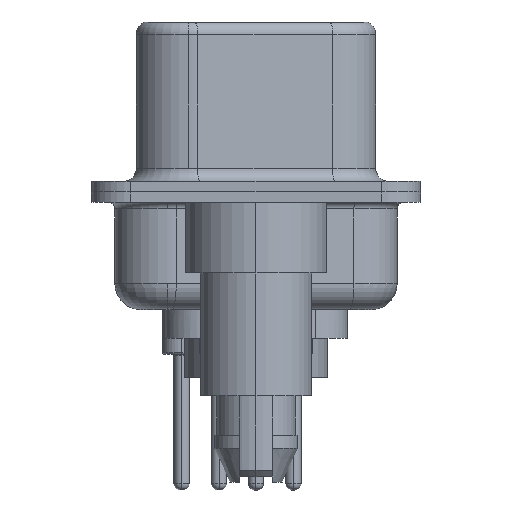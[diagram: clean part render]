
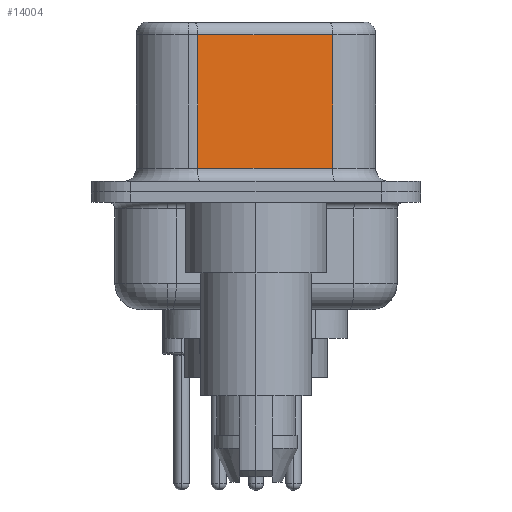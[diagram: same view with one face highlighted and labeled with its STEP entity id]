
A CAD part, left-side view. The second image highlights one B-rep face of the part: STEP entity #14004.
In plain terms, the highlighted planar face has unit normal (-0.985, -0.174, 0).
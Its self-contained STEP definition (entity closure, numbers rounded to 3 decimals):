
#1458 = EDGE_CURVE ( 'NONE', #4819, #14677, #11647, .T. ) ;
#2190 = VERTEX_POINT ( 'NONE', #2467 ) ;
#2467 = CARTESIAN_POINT ( 'NONE',  ( 4.585, -2.927, 0.9 ) ) ;
#2609 = DIRECTION ( 'NONE',  ( -0.174, 0.985, 0. ) ) ;
#2618 = LINE ( 'NONE', #23631, #12493 ) ;
#2813 = EDGE_CURVE ( 'NONE', #15914, #2190, #2618, .T. ) ;
#3540 = VECTOR ( 'NONE', #10122, 1000. ) ;
#4766 = EDGE_CURVE ( 'NONE', #4819, #2190, #15230, .T. ) ;
#4819 = VERTEX_POINT ( 'NONE', #8885 ) ;
#5804 = ORIENTED_EDGE ( 'NONE', *, *, #1458, .T. ) ;
#6627 = LINE ( 'NONE', #10200, #3540 ) ;
#7213 = DIRECTION ( 'NONE',  ( 0.985, 0.174, 0. ) ) ;
#7527 = DIRECTION ( 'NONE',  ( 0.174, -0.985, 0. ) ) ;
#7556 = ORIENTED_EDGE ( 'NONE', *, *, #2813, .T. ) ;
#8885 = CARTESIAN_POINT ( 'NONE',  ( 4.585, -2.927, 6.02 ) ) ;
#9108 = PLANE ( 'NONE',  #25425 ) ;
#9207 = CARTESIAN_POINT ( 'NONE',  ( 4.585, -2.927, 6.52 ) ) ;
#10122 = DIRECTION ( 'NONE',  ( 0., 0., -1. ) ) ;
#10200 = CARTESIAN_POINT ( 'NONE',  ( 3.675, 2.233, 6.52 ) ) ;
#11647 = LINE ( 'NONE', #14417, #18127 ) ;
#12493 = VECTOR ( 'NONE', #7527, 1000. ) ;
#14004 = ADVANCED_FACE ( 'NONE', ( #18443 ), #9108, .F. ) ;
#14287 = CARTESIAN_POINT ( 'NONE',  ( 4.585, -2.927, 6.52 ) ) ;
#14417 = CARTESIAN_POINT ( 'NONE',  ( 4.585, -2.927, 6.02 ) ) ;
#14538 = DIRECTION ( 'NONE',  ( 0., 0., -1. ) ) ;
#14677 = VERTEX_POINT ( 'NONE', #21614 ) ;
#15230 = LINE ( 'NONE', #14287, #24550 ) ;
#15914 = VERTEX_POINT ( 'NONE', #18309 ) ;
#17011 = EDGE_CURVE ( 'NONE', #14677, #15914, #6627, .T. ) ;
#18127 = VECTOR ( 'NONE', #2609, 1000. ) ;
#18309 = CARTESIAN_POINT ( 'NONE',  ( 3.675, 2.233, 0.9 ) ) ;
#18443 = FACE_OUTER_BOUND ( 'NONE', #21652, .T. ) ;
#19085 = DIRECTION ( 'NONE',  ( -0.174, 0.985, 0. ) ) ;
#21564 = ORIENTED_EDGE ( 'NONE', *, *, #4766, .F. ) ;
#21614 = CARTESIAN_POINT ( 'NONE',  ( 3.675, 2.233, 6.02 ) ) ;
#21652 = EDGE_LOOP ( 'NONE', ( #21564, #5804, #22516, #7556 ) ) ;
#22516 = ORIENTED_EDGE ( 'NONE', *, *, #17011, .T. ) ;
#23631 = CARTESIAN_POINT ( 'NONE',  ( 4.585, -2.927, 0.9 ) ) ;
#24550 = VECTOR ( 'NONE', #14538, 1000. ) ;
#25425 = AXIS2_PLACEMENT_3D ( 'NONE', #9207, #7213, #19085 ) ;
